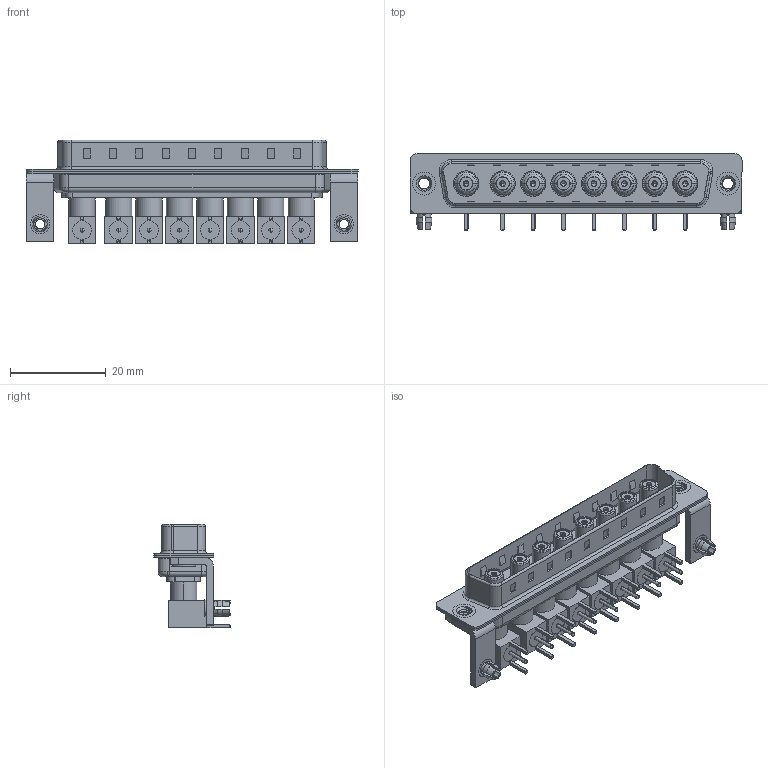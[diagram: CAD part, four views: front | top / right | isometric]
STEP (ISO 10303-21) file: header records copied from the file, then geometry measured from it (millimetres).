
FILE_DESCRIPTION (( 'STEP AP203' ), '1' );
FILE_NAME ('629-8W8-640-5N3.STEP', '2022-05-14T09:43:05', ( '' ), ( '' ), 'SwSTEP 2.0', 'SolidWorks 2020', '' );
FILE_SCHEMA (( 'CONFIG_CONTROL_DESIGN' ));
Length unit declared in the file: millimetre
Products named in the file (22): Co-Ax Jack_RA PC Tail; Socket_RA; 629-8W8-640-5N3; 629Combo Threaded Rivet_3; 629Combo Housing_8W8; Co-Ax Jack Assy_RA; 629Combo Board Lock; Locking Collar; Insulator Socket 2; 629Combo Shell Front_37 Contacts; Insulator Socket; 629Combo Stabilizer Bracket; RA Back Shell; 629Combo Shell Rear_37 Contacts; Insulator RA Pin
Assembly tree (73 placements, depth 3):
  629-8W8-640-5N3
    629Combo Housing_8W8
    629Combo Shell Rear_37 Contacts
    629Combo Shell Front_37 Contacts
    629Combo Threaded Rivet_3  x2
    629Combo Stabilizer Bracket  x2
    629Combo Board Lock  x2
    Co-Ax Jack Assy_RA
      Co-Ax Jack_RA PC Tail
      Insulator Socket
      Insulator Socket 2
      Locking Collar
      Socket_RA
      RA Back Shell
      Insulator RA Pin
    Co-Ax Jack Assy_RA
      Co-Ax Jack_RA PC Tail
      Insulator Socket
      Insulator Socket 2
      Locking Collar
      Socket_RA
      RA Back Shell
      Insulator RA Pin
    Co-Ax Jack Assy_RA
      Co-Ax Jack_RA PC Tail
      Insulator Socket
      Insulator Socket 2
      Locking Collar
      Socket_RA
      RA Back Shell
      Insulator RA Pin
    Co-Ax Jack Assy_RA
      Co-Ax Jack_RA PC Tail
      Insulator Socket
      Insulator Socket 2
      Locking Collar
      Socket_RA
      RA Back Shell
      Insulator RA Pin
    Co-Ax Jack Assy_RA
      Co-Ax Jack_RA PC Tail
      Insulator Socket
      Insulator Socket 2
      Locking Collar
      Socket_RA
      RA Back Shell
      Insulator RA Pin
    Co-Ax Jack Assy_RA
      Co-Ax Jack_RA PC Tail
      Insulator Socket
      Insulator Socket 2
      Locking Collar
      Socket_RA
      RA Back Shell
      Insulator RA Pin
    Co-Ax Jack Assy_RA
      Co-Ax Jack_RA PC Tail
      Insulator Socket
      Insulator Socket 2
      Locking Collar
Bounding box: 69.4 x 16 x 21.71 mm (x, y, z)
Volume: 6365.3 mm3; surface area: 17552.3 mm2
Topology: 65 solids, 65 shells, 1760 faces, 4167 edges, 2600 vertices
Faces by surface type: cylinder 727, plane 727, cone 178, torus 98, sphere 16, bspline 14
Entity records: 24519 total; most frequent: CARTESIAN_POINT 4989, DIRECTION 3516, ORIENTED_EDGE 3136, EDGE_CURVE 1568, AXIS2_PLACEMENT_3D 1303, VERTEX_POINT 996, VECTOR 910, LINE 910
